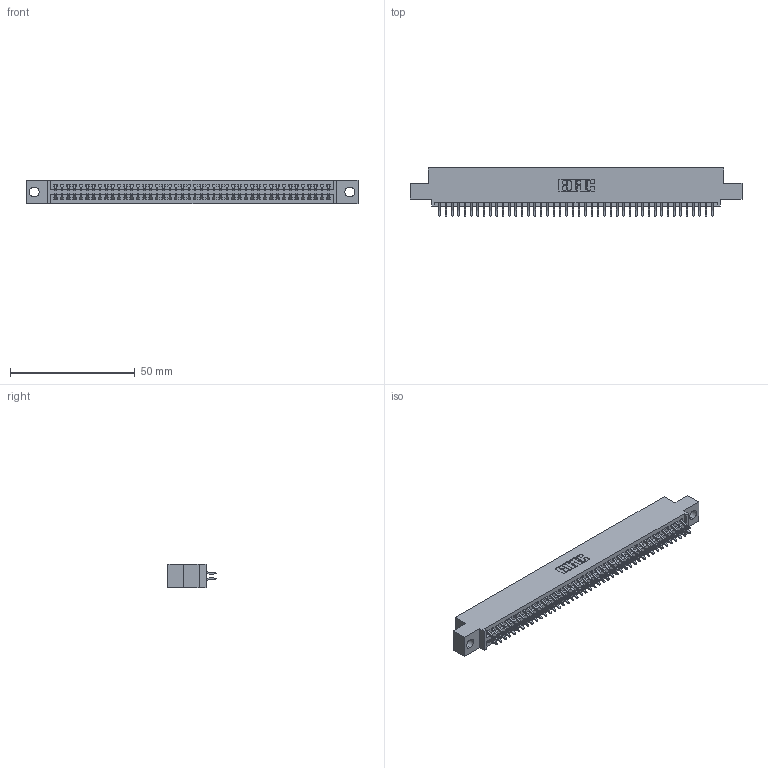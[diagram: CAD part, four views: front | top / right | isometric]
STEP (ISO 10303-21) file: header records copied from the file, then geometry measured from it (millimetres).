
FILE_DESCRIPTION (( 'STEP AP203' ), '1' );
FILE_NAME ('345-088-556-504.STEP', '2018-10-04T14:46:50', ( '' ), ( '' ), 'SwSTEP 2.0', 'SolidWorks 2016', '' );
FILE_SCHEMA (( 'CONFIG_CONTROL_DESIGN' ));
Length unit declared in the file: inch
Products named in the file (3): 345-088-556-504; 345-292-001_556 Tail; 345 Part_0.110 Offset - 0.156 Dia-TH
Assembly tree (89 placements, depth 2):
  345-088-556-504
    345 Part_0.110 Offset - 0.156 Dia-TH
    345-292-001_556 Tail  x88
Bounding box: 132.97 x 19.24 x 9.4 mm (x, y, z)
Volume: 12770.6 mm3; surface area: 18746.8 mm2
Topology: 89 solids, 89 shells, 5058 faces, 15049 edges, 9914 vertices
Faces by surface type: plane 3340, cylinder 1718
Entity records: 34609 total; most frequent: CARTESIAN_POINT 5816, ORIENTED_EDGE 5738, DIRECTION 5113, EDGE_CURVE 2869, VECTOR 2553, LINE 2553, VERTEX_POINT 1910, AXIS2_PLACEMENT_3D 1280
